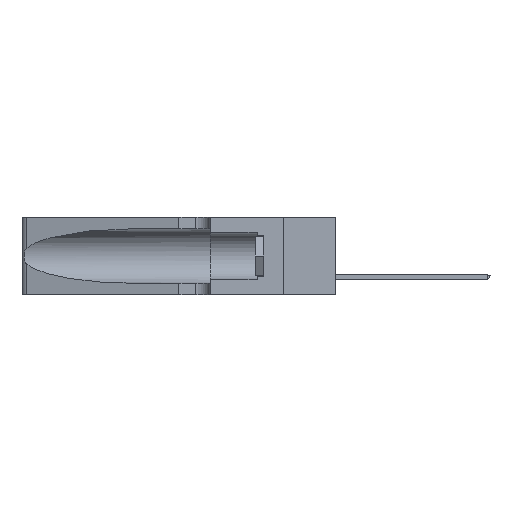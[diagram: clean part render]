
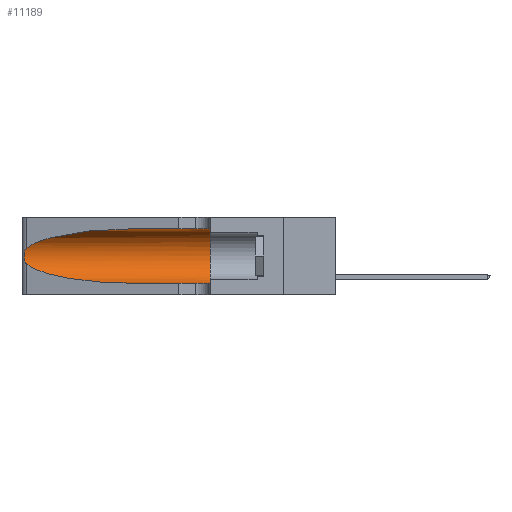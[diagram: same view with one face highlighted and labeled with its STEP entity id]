
A CAD part, left-side view. The second image highlights one B-rep face of the part: STEP entity #11189.
In plain terms, the highlighted cylindrical face has radius 3.308 mm (diameter 6.617 mm), a partial arc.
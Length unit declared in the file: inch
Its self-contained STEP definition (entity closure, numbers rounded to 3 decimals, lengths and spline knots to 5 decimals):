
#252 = CARTESIAN_POINT ( 'NONE',  ( 0.25787, 1.23484, 0.2124 ) ) ;
#527 = VERTEX_POINT ( 'NONE', #1327 ) ;
#1327 = CARTESIAN_POINT ( 'NONE',  ( 0.1305, 0.35, 0.31525 ) ) ;
#1398 = EDGE_LOOP ( 'NONE', ( #21925, #6943, #9124, #1701, #23617, #2331 ) ) ;
#1701 = ORIENTED_EDGE ( 'NONE', *, *, #12738, .T. ) ;
#2331 = ORIENTED_EDGE ( 'NONE', *, *, #10424, .F. ) ;
#2375 = LINE ( 'NONE', #23321, #22097 ) ;
#3969 = CARTESIAN_POINT ( 'NONE',  ( 0.25555, 1.22994, 0.2215 ) ) ;
#4056 = CARTESIAN_POINT ( 'NONE',  ( 0.25487, 1.22718, 0.14631 ) ) ;
#4324 = CARTESIAN_POINT ( 'NONE',  ( 0.26075, 1.23896, 0.19203 ) ) ;
#4611 = CARTESIAN_POINT ( 'NONE',  ( 0.1305, 0.72297, 0.05475 ) ) ;
#4867 = CARTESIAN_POINT ( 'NONE',  ( 0.25487, 1.22718, 0.14631 ) ) ;
#5708 = CARTESIAN_POINT ( 'NONE',  ( 0.1305, 0.35, 0.05475 ) ) ;
#6284 = CARTESIAN_POINT ( 'NONE',  ( 0.1305, 1.61858, 0.05475 ) ) ;
#6943 = ORIENTED_EDGE ( 'NONE', *, *, #17680, .T. ) ;
#7477 = AXIS2_PLACEMENT_3D ( 'NONE', #24644, #20290, #26564 ) ;
#7750 = DIRECTION ( 'NONE',  ( 0., 0., -1. ) ) ;
#9014 = CARTESIAN_POINT ( 'NONE',  ( 0.18966, 0.96281, 0.05475 ) ) ;
#9122 = FACE_OUTER_BOUND ( 'NONE', #1398, .T. ) ;
#9124 = ORIENTED_EDGE ( 'NONE', *, *, #23397, .T. ) ;
#9136 = B_SPLINE_CURVE_WITH_KNOTS ( 'NONE', 3,
 ( #18655, #3969, #22521, #252, #24642, #20463, #4324, #24809, #14498, #12249, #20549, #18571, #10442, #4056 ),
 .UNSPECIFIED., .F., .F.,
 ( 4, 2, 2, 2, 2, 2, 4 ),
 ( 0., 0.00027, 0.00053, 0.00107, 0.0016, 0.00187, 0.00214 ),
 .UNSPECIFIED. ) ;
#9498 = VERTEX_POINT ( 'NONE', #5708 ) ;
#10424 = EDGE_CURVE ( 'NONE', #13926, #527, #2375, .T. ) ;
#10442 = CARTESIAN_POINT ( 'NONE',  ( 0.25555, 1.22993, 0.14849 ) ) ;
#11189 = ADVANCED_FACE ( 'NONE', ( #9122 ), #16843, .F. ) ;
#11408 = CIRCLE ( 'NONE', #7477, 0.13025 ) ;
#11489 = VERTEX_POINT ( 'NONE', #15385 ) ;
#12107 = CARTESIAN_POINT ( 'NONE',  ( 0.25487, 1.22718, 0.22369 ) ) ;
#12187 = CARTESIAN_POINT ( 'NONE',  ( 0.18966, 0.96281, 0.31525 ) ) ;
#12249 = CARTESIAN_POINT ( 'NONE',  ( 0.25856, 1.23593, 0.16098 ) ) ;
#12400 = DIRECTION ( 'NONE',  ( 0., -1., 0. ) ) ;
#12738 = EDGE_CURVE ( 'NONE', #19771, #9498, #18079, .T. ) ;
#13059 = CARTESIAN_POINT ( 'NONE',  ( 0.1305, 0.72297, 0.05475 ) ) ;
#13286 = DIRECTION ( 'NONE',  ( 0., -1., 0. ) ) ;
#13926 = VERTEX_POINT ( 'NONE', #25505 ) ;
#14234 = EDGE_CURVE ( 'NONE', #527, #9498, #11408, .T. ) ;
#14288 = CARTESIAN_POINT ( 'NONE',  ( 0.1305, 1.61858, 0.185 ) ) ;
#14498 = CARTESIAN_POINT ( 'NONE',  ( 0.26017, 1.23833, 0.17102 ) ) ;
#14582 =( BOUNDED_CURVE ( )  B_SPLINE_CURVE ( 3, ( #4867, #23458, #9014, #13059 ),
 .UNSPECIFIED., .F., .F. ) 
 B_SPLINE_CURVE_WITH_KNOTS ( ( 4, 4 ),
 ( 3.44316, 4.71239 ),
 .UNSPECIFIED. ) 
 CURVE ( )  GEOMETRIC_REPRESENTATION_ITEM ( )  RATIONAL_B_SPLINE_CURVE ( ( 1., 0.87, 0.87, 1. ) ) 
 REPRESENTATION_ITEM ( '' )  );
#15369 = AXIS2_PLACEMENT_3D ( 'NONE', #14288, #20339, #7750 ) ;
#15385 = CARTESIAN_POINT ( 'NONE',  ( 0.25487, 1.22718, 0.22369 ) ) ;
#16167 = CARTESIAN_POINT ( 'NONE',  ( 0.2373, 1.15595, 0.28018 ) ) ;
#16843 = CYLINDRICAL_SURFACE ( 'NONE', #15369, 0.13025 ) ;
#17680 = EDGE_CURVE ( 'NONE', #11489, #19467, #9136, .T. ) ;
#18074 = CARTESIAN_POINT ( 'NONE',  ( 0.1305, 0.72297, 0.31525 ) ) ;
#18079 = LINE ( 'NONE', #6284, #19370 ) ;
#18297 = EDGE_CURVE ( 'NONE', #13926, #11489, #23024, .T. ) ;
#18571 = CARTESIAN_POINT ( 'NONE',  ( 0.25639, 1.23186, 0.15144 ) ) ;
#18655 = CARTESIAN_POINT ( 'NONE',  ( 0.25487, 1.22718, 0.22369 ) ) ;
#19370 = VECTOR ( 'NONE', #12400, 39.37008 ) ;
#19467 = VERTEX_POINT ( 'NONE', #25470 ) ;
#19771 = VERTEX_POINT ( 'NONE', #4611 ) ;
#20290 = DIRECTION ( 'NONE',  ( 0., 1., 0. ) ) ;
#20339 = DIRECTION ( 'NONE',  ( 0., -1., 0. ) ) ;
#20463 = CARTESIAN_POINT ( 'NONE',  ( 0.26018, 1.23835, 0.19895 ) ) ;
#20549 = CARTESIAN_POINT ( 'NONE',  ( 0.25789, 1.23486, 0.15765 ) ) ;
#21925 = ORIENTED_EDGE ( 'NONE', *, *, #18297, .T. ) ;
#22097 = VECTOR ( 'NONE', #13286, 39.37008 ) ;
#22521 = CARTESIAN_POINT ( 'NONE',  ( 0.25639, 1.23184, 0.21858 ) ) ;
#23024 =( BOUNDED_CURVE ( )  B_SPLINE_CURVE ( 3, ( #18074, #12187, #16167, #12107 ),
 .UNSPECIFIED., .F., .F. ) 
 B_SPLINE_CURVE_WITH_KNOTS ( ( 4, 4 ),
 ( 1.5708, 2.84003 ),
 .UNSPECIFIED. ) 
 CURVE ( )  GEOMETRIC_REPRESENTATION_ITEM ( )  RATIONAL_B_SPLINE_CURVE ( ( 1., 0.87, 0.87, 1. ) ) 
 REPRESENTATION_ITEM ( '' )  );
#23321 = CARTESIAN_POINT ( 'NONE',  ( 0.1305, 1.61858, 0.31525 ) ) ;
#23397 = EDGE_CURVE ( 'NONE', #19467, #19771, #14582, .T. ) ;
#23458 = CARTESIAN_POINT ( 'NONE',  ( 0.2373, 1.15595, 0.08982 ) ) ;
#23617 = ORIENTED_EDGE ( 'NONE', *, *, #14234, .F. ) ;
#24642 = CARTESIAN_POINT ( 'NONE',  ( 0.25854, 1.2359, 0.20912 ) ) ;
#24644 = CARTESIAN_POINT ( 'NONE',  ( 0.1305, 0.35, 0.185 ) ) ;
#24809 = CARTESIAN_POINT ( 'NONE',  ( 0.26075, 1.23896, 0.178 ) ) ;
#25470 = CARTESIAN_POINT ( 'NONE',  ( 0.25487, 1.22718, 0.14631 ) ) ;
#25505 = CARTESIAN_POINT ( 'NONE',  ( 0.1305, 0.72297, 0.31525 ) ) ;
#26564 = DIRECTION ( 'NONE',  ( 0., 0., 1. ) ) ;
